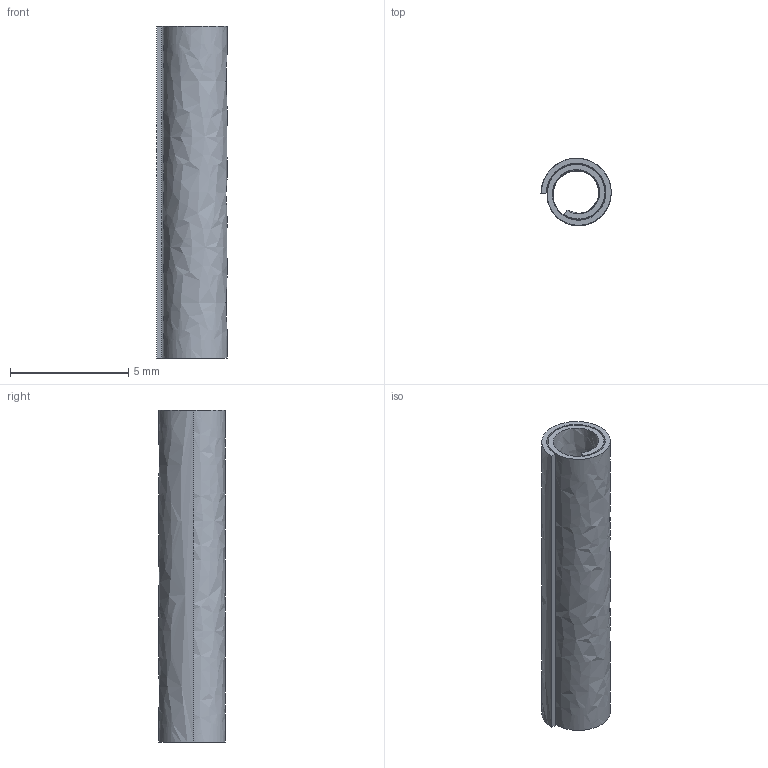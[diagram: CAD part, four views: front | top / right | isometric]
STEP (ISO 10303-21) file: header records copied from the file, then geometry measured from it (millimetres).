
FILE_DESCRIPTION (( 'STEP AP214' ), '1' );
FILE_NAME ('Spring Pin.step', '2014-07-30T19:47:01', ( 'WarFairy' ), ( '' ), 'SwSTEP 2.0', 'SolidWorks 2013', '' );
FILE_SCHEMA (( 'AUTOMOTIVE_DESIGN' ));
Length unit declared in the file: millimetre
Products named in the file (1): Spring Pin
Bounding box: 2.97 x 2.83 x 14.02 mm (x, y, z)
Volume: 41.9 mm3; surface area: 400.2 mm2
Topology: 1 solids, 1 shells, 6 faces, 12 edges, 8 vertices
Faces by surface type: plane 4, bspline 2
Entity records: 386 total; most frequent: CARTESIAN_POINT 237, ORIENTED_EDGE 24, DIRECTION 18, EDGE_CURVE 12, VECTOR 8, LINE 8, VERTEX_POINT 8, FACE_OUTER_BOUND 6
